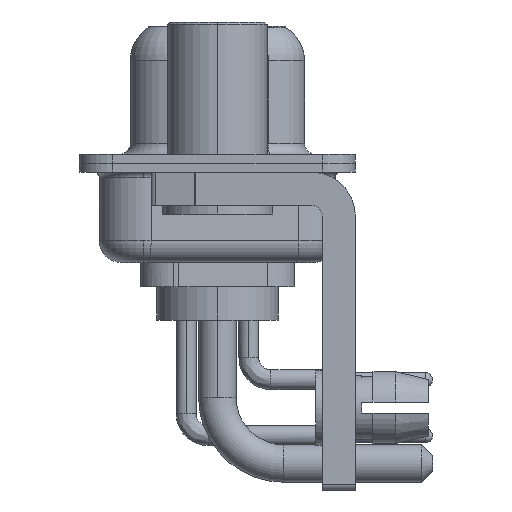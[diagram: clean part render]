
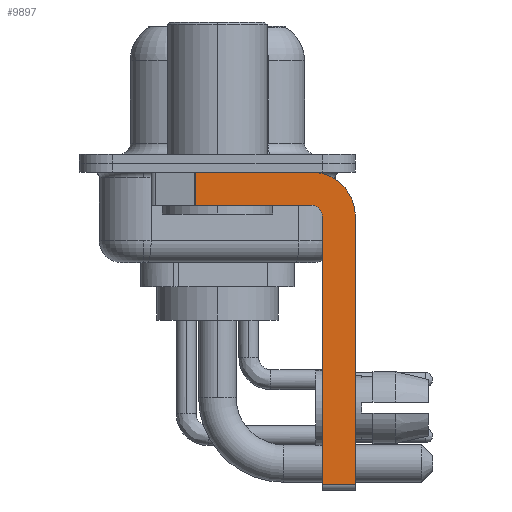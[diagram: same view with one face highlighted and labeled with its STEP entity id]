
A CAD part, left-side view. The second image highlights one B-rep face of the part: STEP entity #9897.
In plain terms, the highlighted planar face has unit normal (-1, 0, 0).
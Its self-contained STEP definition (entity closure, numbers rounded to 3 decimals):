
#210 = CARTESIAN_POINT ( 'NONE',  ( -2.9, -6.25, -2.4 ) ) ;
#476 = LINE ( 'NONE', #6834, #2710 ) ;
#543 = VERTEX_POINT ( 'NONE', #26520 ) ;
#628 = VECTOR ( 'NONE', #9585, 1000. ) ;
#903 = DIRECTION ( 'NONE',  ( 0., 0., 1. ) ) ;
#968 = FACE_OUTER_BOUND ( 'NONE', #5229, .T. ) ;
#1266 = EDGE_CURVE ( 'NONE', #5742, #4414, #17065, .T. ) ;
#1469 = CARTESIAN_POINT ( 'NONE',  ( -2.9, -4.25, -2.4 ) ) ;
#1691 = VECTOR ( 'NONE', #17083, 1000. ) ;
#2173 = CARTESIAN_POINT ( 'NONE',  ( -2.9, -4.75, -14.8 ) ) ;
#2652 = DIRECTION ( 'NONE',  ( 0., -1., 0. ) ) ;
#2710 = VECTOR ( 'NONE', #23306, 1000. ) ;
#3124 = CARTESIAN_POINT ( 'NONE',  ( -2.9, -4.25, -0.4 ) ) ;
#3497 = VERTEX_POINT ( 'NONE', #18981 ) ;
#4414 = VERTEX_POINT ( 'NONE', #24995 ) ;
#4463 = CIRCLE ( 'NONE', #26996, 2. ) ;
#4932 = VERTEX_POINT ( 'NONE', #27284 ) ;
#5229 = EDGE_LOOP ( 'NONE', ( #23888, #14442, #18907, #19839, #11242, #24472, #23930, #7582 ) ) ;
#5493 = EDGE_CURVE ( 'NONE', #18158, #26651, #4463, .T. ) ;
#5742 = VERTEX_POINT ( 'NONE', #15581 ) ;
#6075 = EDGE_CURVE ( 'NONE', #3497, #543, #476, .T. ) ;
#6237 = CARTESIAN_POINT ( 'NONE',  ( -2.9, -4.25, -1.9 ) ) ;
#6834 = CARTESIAN_POINT ( 'NONE',  ( -2.9, -4.25, -14.55 ) ) ;
#6966 = EDGE_CURVE ( 'NONE', #4932, #4414, #13016, .T. ) ;
#6995 = CARTESIAN_POINT ( 'NONE',  ( -2.9, -4.25, -2.4 ) ) ;
#7582 = ORIENTED_EDGE ( 'NONE', *, *, #5493, .F. ) ;
#7836 = DIRECTION ( 'NONE',  ( 1., 0., 0. ) ) ;
#8180 = DIRECTION ( 'NONE',  ( 0., 1., 0. ) ) ;
#9585 = DIRECTION ( 'NONE',  ( 0., 0., -1. ) ) ;
#9803 = VERTEX_POINT ( 'NONE', #23793 ) ;
#9897 = ADVANCED_FACE ( 'NONE', ( #968 ), #17845, .F. ) ;
#10178 = EDGE_CURVE ( 'NONE', #9803, #4932, #25819, .T. ) ;
#10599 = LINE ( 'NONE', #2173, #13849 ) ;
#10826 = VECTOR ( 'NONE', #2652, 1000. ) ;
#10836 = EDGE_CURVE ( 'NONE', #5742, #18158, #13040, .T. ) ;
#10850 = CARTESIAN_POINT ( 'NONE',  ( -2.9, 0.978, -1.9 ) ) ;
#11242 = ORIENTED_EDGE ( 'NONE', *, *, #22655, .F. ) ;
#13016 = LINE ( 'NONE', #6237, #18202 ) ;
#13040 = LINE ( 'NONE', #21859, #10826 ) ;
#13849 = VECTOR ( 'NONE', #21103, 1000. ) ;
#14442 = ORIENTED_EDGE ( 'NONE', *, *, #1266, .T. ) ;
#15239 = EDGE_CURVE ( 'NONE', #26651, #543, #25120, .T. ) ;
#15581 = CARTESIAN_POINT ( 'NONE',  ( -2.9, 0.978, -0.4 ) ) ;
#15707 = DIRECTION ( 'NONE',  ( -1., 0., 0. ) ) ;
#15947 = CARTESIAN_POINT ( 'NONE',  ( -2.9, -6.25, -2.4 ) ) ;
#17065 = LINE ( 'NONE', #10850, #628 ) ;
#17083 = DIRECTION ( 'NONE',  ( 0., 0., -1. ) ) ;
#17387 = AXIS2_PLACEMENT_3D ( 'NONE', #26694, #20459, #22124 ) ;
#17845 = PLANE ( 'NONE',  #17387 ) ;
#18158 = VERTEX_POINT ( 'NONE', #3124 ) ;
#18202 = VECTOR ( 'NONE', #8180, 1000. ) ;
#18907 = ORIENTED_EDGE ( 'NONE', *, *, #6966, .F. ) ;
#18981 = CARTESIAN_POINT ( 'NONE',  ( -2.9, -4.75, -14.55 ) ) ;
#19839 = ORIENTED_EDGE ( 'NONE', *, *, #10178, .F. ) ;
#20459 = DIRECTION ( 'NONE',  ( 1., 0., 0. ) ) ;
#20950 = AXIS2_PLACEMENT_3D ( 'NONE', #6995, #15707, #903 ) ;
#21103 = DIRECTION ( 'NONE',  ( 0., 0., 1. ) ) ;
#21859 = CARTESIAN_POINT ( 'NONE',  ( -2.9, 3., -0.4 ) ) ;
#22124 = DIRECTION ( 'NONE',  ( 0., 0., -1. ) ) ;
#22655 = EDGE_CURVE ( 'NONE', #3497, #9803, #10599, .T. ) ;
#23306 = DIRECTION ( 'NONE',  ( 0., -1., 0. ) ) ;
#23793 = CARTESIAN_POINT ( 'NONE',  ( -2.9, -4.75, -2.4 ) ) ;
#23888 = ORIENTED_EDGE ( 'NONE', *, *, #10836, .F. ) ;
#23930 = ORIENTED_EDGE ( 'NONE', *, *, #15239, .F. ) ;
#24472 = ORIENTED_EDGE ( 'NONE', *, *, #6075, .T. ) ;
#24703 = DIRECTION ( 'NONE',  ( 0., 0., -1. ) ) ;
#24995 = CARTESIAN_POINT ( 'NONE',  ( -2.9, 0.978, -1.9 ) ) ;
#25120 = LINE ( 'NONE', #210, #1691 ) ;
#25819 = CIRCLE ( 'NONE', #20950, 0.5 ) ;
#26520 = CARTESIAN_POINT ( 'NONE',  ( -2.9, -6.25, -14.55 ) ) ;
#26651 = VERTEX_POINT ( 'NONE', #15947 ) ;
#26694 = CARTESIAN_POINT ( 'NONE',  ( -2.9, -4.25, -2.4 ) ) ;
#26996 = AXIS2_PLACEMENT_3D ( 'NONE', #1469, #7836, #24703 ) ;
#27284 = CARTESIAN_POINT ( 'NONE',  ( -2.9, -4.25, -1.9 ) ) ;
